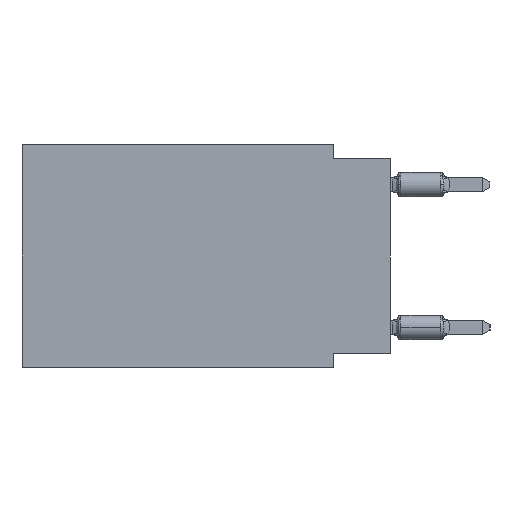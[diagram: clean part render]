
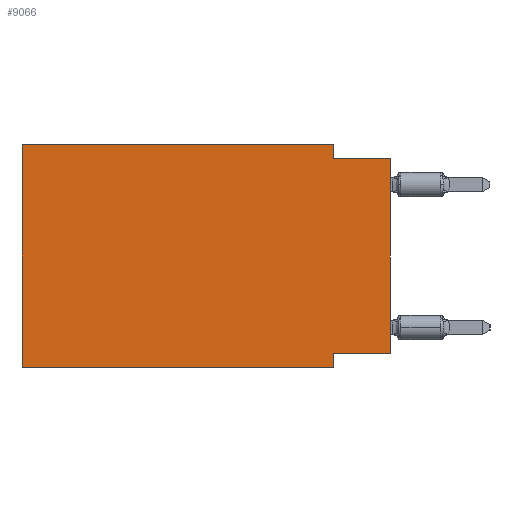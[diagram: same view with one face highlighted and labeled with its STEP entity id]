
A CAD part, left-side view. The second image highlights one B-rep face of the part: STEP entity #9066.
In plain terms, the highlighted planar face has unit normal (-1, 0, 0).
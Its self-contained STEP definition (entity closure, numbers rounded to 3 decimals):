
#207 = CARTESIAN_POINT ( 'NONE',  ( 0., 16.383, 0. ) ) ;
#477 = CARTESIAN_POINT ( 'NONE',  ( 0., 16.383, -9.906 ) ) ;
#1129 = VERTEX_POINT ( 'NONE', #15884 ) ;
#1142 = VERTEX_POINT ( 'NONE', #12611 ) ;
#1464 = AXIS2_PLACEMENT_3D ( 'NONE', #207, #18343, #27229 ) ;
#2288 = CARTESIAN_POINT ( 'NONE',  ( 0., 0., 0. ) ) ;
#2762 = ORIENTED_EDGE ( 'NONE', *, *, #31932, .T. ) ;
#2935 = CARTESIAN_POINT ( 'NONE',  ( 0., 2.54, 0. ) ) ;
#3104 = FACE_OUTER_BOUND ( 'NONE', #5469, .T. ) ;
#3963 = LINE ( 'NONE', #33128, #19951 ) ;
#5173 = LINE ( 'NONE', #2288, #31266 ) ;
#5263 = CARTESIAN_POINT ( 'NONE',  ( 0., 2.54, 0. ) ) ;
#5296 = EDGE_CURVE ( 'NONE', #5344, #37597, #20676, .T. ) ;
#5344 = VERTEX_POINT ( 'NONE', #2935 ) ;
#5469 = EDGE_LOOP ( 'NONE', ( #33676, #23389, #35890, #29256, #22334, #2762, #22076, #16489 ) ) ;
#5708 = VERTEX_POINT ( 'NONE', #29144 ) ;
#6805 = CARTESIAN_POINT ( 'NONE',  ( 0., 16.383, 0. ) ) ;
#7687 = EDGE_CURVE ( 'NONE', #37597, #1129, #3963, .T. ) ;
#8648 = EDGE_CURVE ( 'NONE', #9966, #1142, #14760, .T. ) ;
#9044 = CARTESIAN_POINT ( 'NONE',  ( 0., 16.383, 0. ) ) ;
#9066 = ADVANCED_FACE ( 'NONE', ( #3104 ), #26861, .F. ) ;
#9307 = DIRECTION ( 'NONE',  ( 0., 0., -1. ) ) ;
#9455 = VECTOR ( 'NONE', #9307, 1000. ) ;
#9966 = VERTEX_POINT ( 'NONE', #34033 ) ;
#10431 = VECTOR ( 'NONE', #36024, 1000. ) ;
#12572 = CARTESIAN_POINT ( 'NONE',  ( 0., 2.54, -9.906 ) ) ;
#12611 = CARTESIAN_POINT ( 'NONE',  ( 0., 16.383, 0. ) ) ;
#13572 = VECTOR ( 'NONE', #30382, 1000. ) ;
#14760 = LINE ( 'NONE', #6805, #22377 ) ;
#14948 = VECTOR ( 'NONE', #32992, 1000. ) ;
#15469 = LINE ( 'NONE', #12572, #9455 ) ;
#15780 = VECTOR ( 'NONE', #34997, 1000. ) ;
#15884 = CARTESIAN_POINT ( 'NONE',  ( 0., 0., -0.635 ) ) ;
#16085 = LINE ( 'NONE', #33687, #10431 ) ;
#16489 = ORIENTED_EDGE ( 'NONE', *, *, #37252, .F. ) ;
#18343 = DIRECTION ( 'NONE',  ( 1., 0., 0. ) ) ;
#19345 = VERTEX_POINT ( 'NONE', #31518 ) ;
#19951 = VECTOR ( 'NONE', #27523, 1000. ) ;
#20676 = LINE ( 'NONE', #5263, #15780 ) ;
#21747 = EDGE_CURVE ( 'NONE', #5708, #28964, #15469, .T. ) ;
#22076 = ORIENTED_EDGE ( 'NONE', *, *, #21747, .F. ) ;
#22334 = ORIENTED_EDGE ( 'NONE', *, *, #8648, .F. ) ;
#22377 = VECTOR ( 'NONE', #29270, 1000. ) ;
#23389 = ORIENTED_EDGE ( 'NONE', *, *, #7687, .F. ) ;
#24222 = LINE ( 'NONE', #477, #13572 ) ;
#24649 = EDGE_CURVE ( 'NONE', #1142, #5344, #29503, .T. ) ;
#26861 = PLANE ( 'NONE',  #1464 ) ;
#27229 = DIRECTION ( 'NONE',  ( 0., 0., -1. ) ) ;
#27523 = DIRECTION ( 'NONE',  ( 0., -1., 0. ) ) ;
#28964 = VERTEX_POINT ( 'NONE', #33990 ) ;
#29144 = CARTESIAN_POINT ( 'NONE',  ( 0., 2.54, -9.271 ) ) ;
#29256 = ORIENTED_EDGE ( 'NONE', *, *, #24649, .F. ) ;
#29270 = DIRECTION ( 'NONE',  ( 0., 0., 1. ) ) ;
#29503 = LINE ( 'NONE', #9044, #14948 ) ;
#29550 = EDGE_CURVE ( 'NONE', #19345, #1129, #5173, .T. ) ;
#30382 = DIRECTION ( 'NONE',  ( 0., -1., 0. ) ) ;
#31266 = VECTOR ( 'NONE', #31430, 1000. ) ;
#31430 = DIRECTION ( 'NONE',  ( 0., 0., 1. ) ) ;
#31518 = CARTESIAN_POINT ( 'NONE',  ( 0., 0., -9.271 ) ) ;
#31932 = EDGE_CURVE ( 'NONE', #9966, #28964, #24222, .T. ) ;
#32992 = DIRECTION ( 'NONE',  ( 0., -1., 0. ) ) ;
#33128 = CARTESIAN_POINT ( 'NONE',  ( 0., 0., -0.635 ) ) ;
#33676 = ORIENTED_EDGE ( 'NONE', *, *, #29550, .T. ) ;
#33687 = CARTESIAN_POINT ( 'NONE',  ( 0., 0., -9.271 ) ) ;
#33990 = CARTESIAN_POINT ( 'NONE',  ( 0., 2.54, -9.906 ) ) ;
#34033 = CARTESIAN_POINT ( 'NONE',  ( 0., 16.383, -9.906 ) ) ;
#34997 = DIRECTION ( 'NONE',  ( 0., 0., -1. ) ) ;
#35203 = CARTESIAN_POINT ( 'NONE',  ( 0., 2.54, -0.635 ) ) ;
#35890 = ORIENTED_EDGE ( 'NONE', *, *, #5296, .F. ) ;
#36024 = DIRECTION ( 'NONE',  ( 0., 1., 0. ) ) ;
#37252 = EDGE_CURVE ( 'NONE', #19345, #5708, #16085, .T. ) ;
#37597 = VERTEX_POINT ( 'NONE', #35203 ) ;
